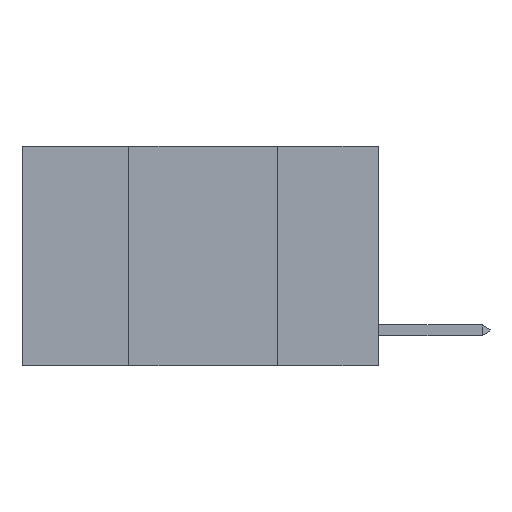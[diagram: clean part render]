
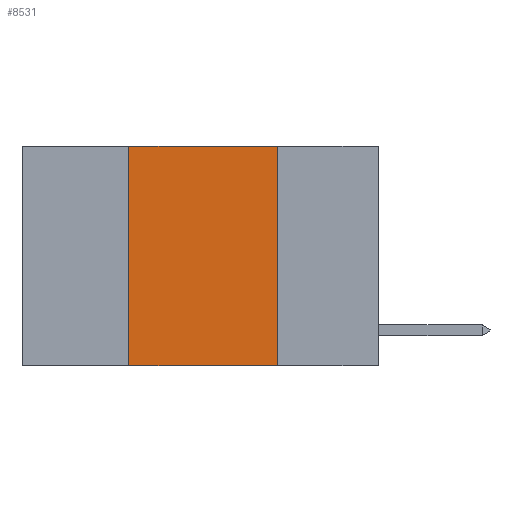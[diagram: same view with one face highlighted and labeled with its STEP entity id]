
A CAD part, left-side view. The second image highlights one B-rep face of the part: STEP entity #8531.
In plain terms, the highlighted planar face has unit normal (-1, 0, 0).
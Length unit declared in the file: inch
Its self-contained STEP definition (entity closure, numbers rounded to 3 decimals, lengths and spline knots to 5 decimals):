
#483 = DIRECTION ( 'NONE',  ( 1., 0., 0. ) ) ;
#761 = VERTEX_POINT ( 'NONE', #12917 ) ;
#781 = LINE ( 'NONE', #10743, #8888 ) ;
#948 = ORIENTED_EDGE ( 'NONE', *, *, #3918, .F. ) ;
#1363 = VECTOR ( 'NONE', #6488, 39.37008 ) ;
#1511 = VECTOR ( 'NONE', #2963, 39.37008 ) ;
#2329 = CARTESIAN_POINT ( 'NONE',  ( 0., 0.17, 0. ) ) ;
#2500 = EDGE_CURVE ( 'NONE', #4614, #3355, #6995, .T. ) ;
#2963 = DIRECTION ( 'NONE',  ( 0., 0., -1. ) ) ;
#3278 = CARTESIAN_POINT ( 'NONE',  ( 0., 0.6, 0. ) ) ;
#3355 = VERTEX_POINT ( 'NONE', #10622 ) ;
#3450 = CARTESIAN_POINT ( 'NONE',  ( 0., 0.6, -0.37 ) ) ;
#3556 = DIRECTION ( 'NONE',  ( 0., -1., 0. ) ) ;
#3605 = EDGE_LOOP ( 'NONE', ( #948, #11200, #12823, #3949 ) ) ;
#3738 = EDGE_CURVE ( 'NONE', #761, #13435, #8608, .T. ) ;
#3918 = EDGE_CURVE ( 'NONE', #13435, #3355, #9311, .T. ) ;
#3949 = ORIENTED_EDGE ( 'NONE', *, *, #2500, .T. ) ;
#4468 = DIRECTION ( 'NONE',  ( 0., 0., 1. ) ) ;
#4614 = VERTEX_POINT ( 'NONE', #8361 ) ;
#6144 = AXIS2_PLACEMENT_3D ( 'NONE', #6839, #483, #7912 ) ;
#6284 = EDGE_CURVE ( 'NONE', #4614, #761, #781, .T. ) ;
#6474 = VECTOR ( 'NONE', #3556, 39.37008 ) ;
#6488 = DIRECTION ( 'NONE',  ( 0., -1., 0. ) ) ;
#6839 = CARTESIAN_POINT ( 'NONE',  ( 0., 0.6, 0. ) ) ;
#6995 = LINE ( 'NONE', #3450, #1363 ) ;
#7912 = DIRECTION ( 'NONE',  ( 0., 0., -1. ) ) ;
#8361 = CARTESIAN_POINT ( 'NONE',  ( 0., 0.42, -0.37 ) ) ;
#8531 = ADVANCED_FACE ( 'NONE', ( #10315 ), #12095, .F. ) ;
#8608 = LINE ( 'NONE', #3278, #6474 ) ;
#8888 = VECTOR ( 'NONE', #4468, 39.37008 ) ;
#9311 = LINE ( 'NONE', #2329, #1511 ) ;
#10315 = FACE_OUTER_BOUND ( 'NONE', #3605, .T. ) ;
#10622 = CARTESIAN_POINT ( 'NONE',  ( 0., 0.17, -0.37 ) ) ;
#10743 = CARTESIAN_POINT ( 'NONE',  ( 0., 0.42, 0. ) ) ;
#11200 = ORIENTED_EDGE ( 'NONE', *, *, #3738, .F. ) ;
#12095 = PLANE ( 'NONE',  #6144 ) ;
#12492 = CARTESIAN_POINT ( 'NONE',  ( 0., 0.17, 0. ) ) ;
#12823 = ORIENTED_EDGE ( 'NONE', *, *, #6284, .F. ) ;
#12917 = CARTESIAN_POINT ( 'NONE',  ( 0., 0.42, 0. ) ) ;
#13435 = VERTEX_POINT ( 'NONE', #12492 ) ;
